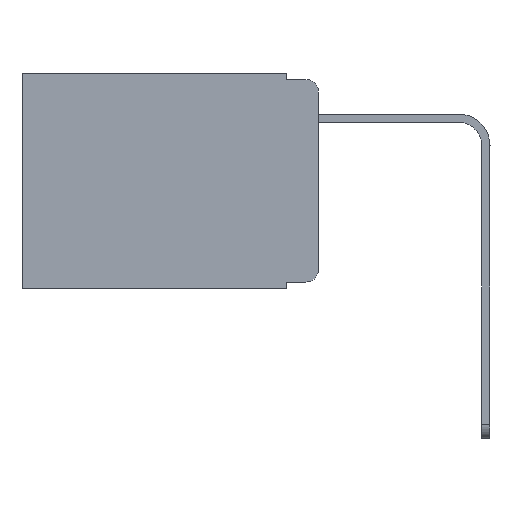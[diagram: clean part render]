
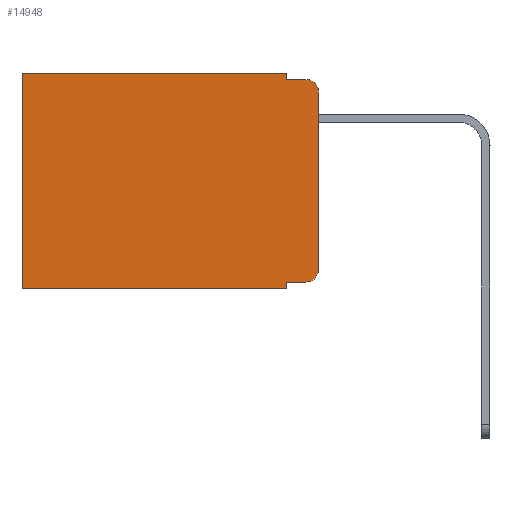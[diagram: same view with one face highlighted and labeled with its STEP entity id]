
A CAD part, left-side view. The second image highlights one B-rep face of the part: STEP entity #14948.
In plain terms, the highlighted planar face has unit normal (-1, 0, 0).
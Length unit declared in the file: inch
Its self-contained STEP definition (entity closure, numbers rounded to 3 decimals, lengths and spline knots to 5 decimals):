
#251 = VECTOR ( 'NONE', #4410, 39.37008 ) ;
#390 = DIRECTION ( 'NONE',  ( 0., 1., 0. ) ) ;
#572 = CARTESIAN_POINT ( 'NONE',  ( 0.298, 0.02, -0.313 ) ) ;
#595 = LINE ( 'NONE', #2885, #12603 ) ;
#794 = AXIS2_PLACEMENT_3D ( 'NONE', #8232, #9577, #10948 ) ;
#853 = CARTESIAN_POINT ( 'NONE',  ( 0.298, 0.051, 0. ) ) ;
#875 = VERTEX_POINT ( 'NONE', #3277 ) ;
#1104 = CIRCLE ( 'NONE', #15743, 0.02 ) ;
#1189 = CARTESIAN_POINT ( 'NONE',  ( 0.298, 0.051, -0.343 ) ) ;
#1603 = EDGE_CURVE ( 'NONE', #9242, #13338, #1104, .T. ) ;
#1758 = CARTESIAN_POINT ( 'NONE',  ( 0.298, 0., -0.03 ) ) ;
#2165 = ORIENTED_EDGE ( 'NONE', *, *, #4546, .T. ) ;
#2625 = ORIENTED_EDGE ( 'NONE', *, *, #11864, .F. ) ;
#2885 = CARTESIAN_POINT ( 'NONE',  ( 0.298, 0., 0. ) ) ;
#3064 = VERTEX_POINT ( 'NONE', #13828 ) ;
#3277 = CARTESIAN_POINT ( 'NONE',  ( 0.298, 0.473, -0.343 ) ) ;
#3284 = EDGE_CURVE ( 'NONE', #15830, #3064, #13279, .T. ) ;
#3395 = DIRECTION ( 'NONE',  ( 0., 0., -1. ) ) ;
#3509 = CARTESIAN_POINT ( 'NONE',  ( 0.298, 0.051, -0.333 ) ) ;
#3702 = DIRECTION ( 'NONE',  ( 0., 0., -1. ) ) ;
#3709 = EDGE_LOOP ( 'NONE', ( #16692, #16420, #2625, #8135, #13406, #2165, #11442, #10446, #16371, #16910 ) ) ;
#3990 = LINE ( 'NONE', #9464, #13043 ) ;
#4315 = EDGE_CURVE ( 'NONE', #15344, #13338, #11550, .T. ) ;
#4363 = LINE ( 'NONE', #6169, #10269 ) ;
#4387 = CIRCLE ( 'NONE', #5776, 0.02 ) ;
#4410 = DIRECTION ( 'NONE',  ( 0., -1., 0. ) ) ;
#4546 = EDGE_CURVE ( 'NONE', #10648, #875, #16179, .T. ) ;
#4696 = VERTEX_POINT ( 'NONE', #1189 ) ;
#4973 = CARTESIAN_POINT ( 'NONE',  ( 0.298, 0., -0.313 ) ) ;
#5411 = VECTOR ( 'NONE', #3702, 39.37008 ) ;
#5776 = AXIS2_PLACEMENT_3D ( 'NONE', #11012, #9769, #8365 ) ;
#6169 = CARTESIAN_POINT ( 'NONE',  ( 0.298, 0.051, -0.333 ) ) ;
#6431 = VECTOR ( 'NONE', #10180, 39.37008 ) ;
#6540 = EDGE_CURVE ( 'NONE', #15830, #10648, #595, .T. ) ;
#6543 = EDGE_CURVE ( 'NONE', #15344, #9679, #4387, .T. ) ;
#6684 = CARTESIAN_POINT ( 'NONE',  ( 0.298, 0.02, -0.333 ) ) ;
#7570 = DIRECTION ( 'NONE',  ( 0., 0., -1. ) ) ;
#7808 = EDGE_CURVE ( 'NONE', #13443, #9242, #4363, .T. ) ;
#7837 = LINE ( 'NONE', #12385, #251 ) ;
#8095 = CARTESIAN_POINT ( 'NONE',  ( 0.298, 0.051, 0. ) ) ;
#8135 = ORIENTED_EDGE ( 'NONE', *, *, #3284, .F. ) ;
#8232 = CARTESIAN_POINT ( 'NONE',  ( 0.298, 0., 0. ) ) ;
#8365 = DIRECTION ( 'NONE',  ( 0., 0., -1. ) ) ;
#8785 = DIRECTION ( 'NONE',  ( -1., 0., 0. ) ) ;
#8834 = CARTESIAN_POINT ( 'NONE',  ( 0.298, 0.051, 0. ) ) ;
#9150 = EDGE_CURVE ( 'NONE', #13443, #4696, #16554, .T. ) ;
#9168 = DIRECTION ( 'NONE',  ( 0., 1., 0. ) ) ;
#9242 = VERTEX_POINT ( 'NONE', #6684 ) ;
#9447 = VECTOR ( 'NONE', #13732, 39.37008 ) ;
#9464 = CARTESIAN_POINT ( 'NONE',  ( 0.298, 0., -0.343 ) ) ;
#9577 = DIRECTION ( 'NONE',  ( 1., 0., 0. ) ) ;
#9637 = PLANE ( 'NONE',  #794 ) ;
#9679 = VERTEX_POINT ( 'NONE', #17188 ) ;
#9698 = VECTOR ( 'NONE', #7570, 39.37008 ) ;
#9769 = DIRECTION ( 'NONE',  ( -1., 0., 0. ) ) ;
#10180 = DIRECTION ( 'NONE',  ( 0., 0., -1. ) ) ;
#10269 = VECTOR ( 'NONE', #15780, 39.37008 ) ;
#10446 = ORIENTED_EDGE ( 'NONE', *, *, #9150, .F. ) ;
#10532 = CARTESIAN_POINT ( 'NONE',  ( 0.298, 0.473, 0. ) ) ;
#10648 = VERTEX_POINT ( 'NONE', #12297 ) ;
#10948 = DIRECTION ( 'NONE',  ( 0., 0., -1. ) ) ;
#11012 = CARTESIAN_POINT ( 'NONE',  ( 0.298, 0.02, -0.03 ) ) ;
#11442 = ORIENTED_EDGE ( 'NONE', *, *, #12899, .F. ) ;
#11550 = LINE ( 'NONE', #12652, #9447 ) ;
#11864 = EDGE_CURVE ( 'NONE', #3064, #9679, #7837, .T. ) ;
#12297 = CARTESIAN_POINT ( 'NONE',  ( 0.298, 0.473, 0. ) ) ;
#12385 = CARTESIAN_POINT ( 'NONE',  ( 0.298, 0.051, -0.01 ) ) ;
#12603 = VECTOR ( 'NONE', #390, 39.37008 ) ;
#12652 = CARTESIAN_POINT ( 'NONE',  ( 0.298, 0., 0. ) ) ;
#12899 = EDGE_CURVE ( 'NONE', #4696, #875, #3990, .T. ) ;
#13043 = VECTOR ( 'NONE', #9168, 39.37008 ) ;
#13279 = LINE ( 'NONE', #853, #9698 ) ;
#13338 = VERTEX_POINT ( 'NONE', #4973 ) ;
#13406 = ORIENTED_EDGE ( 'NONE', *, *, #6540, .T. ) ;
#13443 = VERTEX_POINT ( 'NONE', #3509 ) ;
#13593 = FACE_OUTER_BOUND ( 'NONE', #3709, .T. ) ;
#13732 = DIRECTION ( 'NONE',  ( 0., 0., -1. ) ) ;
#13828 = CARTESIAN_POINT ( 'NONE',  ( 0.298, 0.051, -0.01 ) ) ;
#14948 = ADVANCED_FACE ( 'NONE', ( #13593 ), #9637, .F. ) ;
#15344 = VERTEX_POINT ( 'NONE', #1758 ) ;
#15743 = AXIS2_PLACEMENT_3D ( 'NONE', #572, #8785, #3395 ) ;
#15780 = DIRECTION ( 'NONE',  ( 0., -1., 0. ) ) ;
#15830 = VERTEX_POINT ( 'NONE', #8095 ) ;
#16179 = LINE ( 'NONE', #10532, #5411 ) ;
#16371 = ORIENTED_EDGE ( 'NONE', *, *, #7808, .T. ) ;
#16420 = ORIENTED_EDGE ( 'NONE', *, *, #6543, .T. ) ;
#16554 = LINE ( 'NONE', #8834, #6431 ) ;
#16692 = ORIENTED_EDGE ( 'NONE', *, *, #4315, .F. ) ;
#16910 = ORIENTED_EDGE ( 'NONE', *, *, #1603, .T. ) ;
#17188 = CARTESIAN_POINT ( 'NONE',  ( 0.298, 0.02, -0.01 ) ) ;
